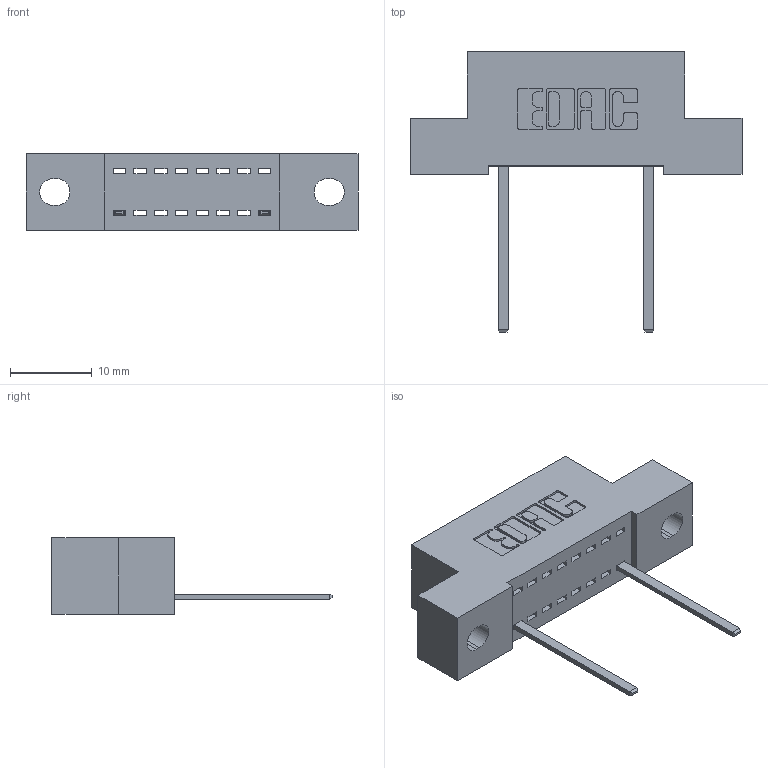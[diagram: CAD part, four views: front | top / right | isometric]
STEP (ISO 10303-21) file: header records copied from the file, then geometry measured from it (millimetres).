
FILE_DESCRIPTION (( 'STEP AP203' ), '1' );
FILE_NAME ('392-008-544-102.STEP', '2018-08-14T19:26:25', ( '' ), ( '' ), 'SwSTEP 2.0', 'SolidWorks 2016', '' );
FILE_SCHEMA (( 'CONFIG_CONTROL_DESIGN' ));
Length unit declared in the file: inch
Products named in the file (3): 342 Part_.128 Slot; 345-292-001_345-293-144; 392-008-544-102
Assembly tree (3 placements, depth 2):
  392-008-544-102
    342 Part_.128 Slot
    345-292-001_345-293-144  x2
Bounding box: 40.64 x 34.3 x 9.4 mm (x, y, z)
Volume: 3340.5 mm3; surface area: 3740.5 mm2
Topology: 3 solids, 3 shells, 290 faces, 879 edges, 582 vertices
Faces by surface type: plane 218, cylinder 72
Entity records: 8915 total; most frequent: CARTESIAN_POINT 1576, ORIENTED_EDGE 1526, DIRECTION 1387, EDGE_CURVE 763, LINE 639, VECTOR 639, VERTEX_POINT 506, AXIS2_PLACEMENT_3D 374
